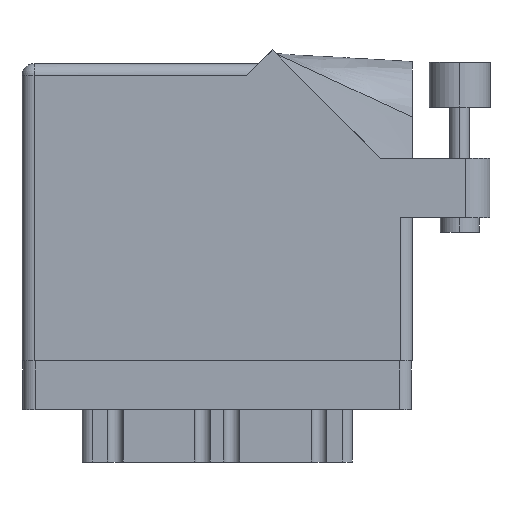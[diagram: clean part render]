
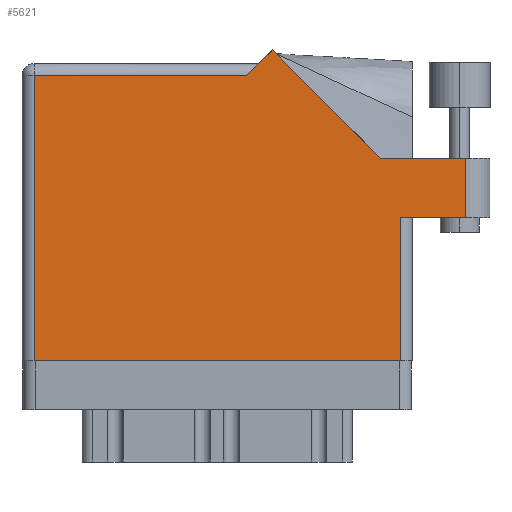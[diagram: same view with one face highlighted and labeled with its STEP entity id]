
A CAD part, front view. The second image highlights one B-rep face of the part: STEP entity #5621.
In plain terms, the highlighted face is planar.
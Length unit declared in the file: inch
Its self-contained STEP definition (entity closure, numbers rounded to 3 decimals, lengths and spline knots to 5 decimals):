
#240 = EDGE_CURVE ( 'NONE', #29193, #4980, #17073, .T. ) ;
#394 = EDGE_CURVE ( 'NONE', #23292, #6392, #9847, .T. ) ;
#606 = VERTEX_POINT ( 'NONE', #11222 ) ;
#652 = DIRECTION ( 'NONE',  ( 0., -1., 0. ) ) ;
#1379 = VECTOR ( 'NONE', #17937, 39.37008 ) ;
#1610 = DIRECTION ( 'NONE',  ( -1., 0., 0. ) ) ;
#2080 = CARTESIAN_POINT ( 'NONE',  ( 1.28771, 1.60071, 0. ) ) ;
#2123 = CARTESIAN_POINT ( 'NONE',  ( 0., 1.468, 0. ) ) ;
#2800 = ORIENTED_EDGE ( 'NONE', *, *, #3490, .T. ) ;
#3029 = ORIENTED_EDGE ( 'NONE', *, *, #5789, .T. ) ;
#3490 = EDGE_CURVE ( 'NONE', #606, #23292, #8045, .T. ) ;
#4129 = VERTEX_POINT ( 'NONE', #16466 ) ;
#4789 = CARTESIAN_POINT ( 'NONE',  ( 0., 1.53, 0. ) ) ;
#4980 = VERTEX_POINT ( 'NONE', #5910 ) ;
#5215 = CARTESIAN_POINT ( 'NONE',  ( 2.285, 1.044, 0. ) ) ;
#5621 = ADVANCED_FACE ( 'NONE', ( #32142 ), #34264, .F. ) ;
#5724 = EDGE_CURVE ( 'NONE', #6392, #8947, #15922, .T. ) ;
#5789 = EDGE_CURVE ( 'NONE', #26999, #606, #16603, .T. ) ;
#5910 = CARTESIAN_POINT ( 'NONE',  ( 1.948, 0., 0. ) ) ;
#6138 = EDGE_CURVE ( 'NONE', #4980, #26999, #32280, .T. ) ;
#6392 = VERTEX_POINT ( 'NONE', #25359 ) ;
#6677 = CARTESIAN_POINT ( 'NONE',  ( 2.285, 1.044, 0. ) ) ;
#7183 = CARTESIAN_POINT ( 'NONE',  ( 2.41, 1.044, 0. ) ) ;
#8045 = LINE ( 'NONE', #5215, #26473 ) ;
#8100 = DIRECTION ( 'NONE',  ( 0., 1., 0. ) ) ;
#8370 = ORIENTED_EDGE ( 'NONE', *, *, #6138, .T. ) ;
#8484 = CARTESIAN_POINT ( 'NONE',  ( 1.84442, 1.044, 0. ) ) ;
#8761 = VECTOR ( 'NONE', #8100, 39.37008 ) ;
#8947 = VERTEX_POINT ( 'NONE', #2080 ) ;
#9288 = CARTESIAN_POINT ( 'NONE',  ( 1.948, 0.737, 0. ) ) ;
#9847 = LINE ( 'NONE', #7183, #1379 ) ;
#10406 = VERTEX_POINT ( 'NONE', #27486 ) ;
#11044 = DIRECTION ( 'NONE',  ( 0., 1., 0. ) ) ;
#11222 = CARTESIAN_POINT ( 'NONE',  ( 2.285, 0.737, 0. ) ) ;
#11412 = LINE ( 'NONE', #21975, #34405 ) ;
#12050 = ORIENTED_EDGE ( 'NONE', *, *, #19920, .T. ) ;
#12279 = EDGE_LOOP ( 'NONE', ( #3029, #2800, #31864, #31094, #23018, #12050, #18805, #20165, #8370 ) ) ;
#12758 = LINE ( 'NONE', #2123, #33790 ) ;
#13274 = CARTESIAN_POINT ( 'NONE',  ( 0., 0., 0. ) ) ;
#13916 = LINE ( 'NONE', #32779, #26219 ) ;
#14462 = AXIS2_PLACEMENT_3D ( 'NONE', #4789, #16093, #34450 ) ;
#15922 = LINE ( 'NONE', #8484, #17833 ) ;
#16093 = DIRECTION ( 'NONE',  ( 0., 0., -1. ) ) ;
#16466 = CARTESIAN_POINT ( 'NONE',  ( 1.155, 1.468, 0. ) ) ;
#16603 = LINE ( 'NONE', #27521, #20105 ) ;
#16894 = DIRECTION ( 'NONE',  ( 1., 0., 0. ) ) ;
#17073 = LINE ( 'NONE', #13274, #17742 ) ;
#17742 = VECTOR ( 'NONE', #16894, 39.37008 ) ;
#17833 = VECTOR ( 'NONE', #30179, 39.37008 ) ;
#17937 = DIRECTION ( 'NONE',  ( -1., 0., 0. ) ) ;
#18805 = ORIENTED_EDGE ( 'NONE', *, *, #31655, .T. ) ;
#19920 = EDGE_CURVE ( 'NONE', #4129, #10406, #12758, .T. ) ;
#20105 = VECTOR ( 'NONE', #22066, 39.37008 ) ;
#20165 = ORIENTED_EDGE ( 'NONE', *, *, #240, .T. ) ;
#21975 = CARTESIAN_POINT ( 'NONE',  ( 1.217, 1.53, 0. ) ) ;
#22066 = DIRECTION ( 'NONE',  ( 1., 0., 0. ) ) ;
#23018 = ORIENTED_EDGE ( 'NONE', *, *, #25516, .T. ) ;
#23292 = VERTEX_POINT ( 'NONE', #6677 ) ;
#23462 = CARTESIAN_POINT ( 'NONE',  ( 1.948, 0.737, 0. ) ) ;
#24282 = DIRECTION ( 'NONE',  ( -0.707, -0.707, 0. ) ) ;
#25359 = CARTESIAN_POINT ( 'NONE',  ( 1.84442, 1.044, 0. ) ) ;
#25516 = EDGE_CURVE ( 'NONE', #8947, #4129, #11412, .T. ) ;
#26219 = VECTOR ( 'NONE', #652, 39.37008 ) ;
#26473 = VECTOR ( 'NONE', #11044, 39.37008 ) ;
#26999 = VERTEX_POINT ( 'NONE', #9288 ) ;
#27486 = CARTESIAN_POINT ( 'NONE',  ( 0.062, 1.468, 0. ) ) ;
#27521 = CARTESIAN_POINT ( 'NONE',  ( 2.01, 0.737, 0. ) ) ;
#29193 = VERTEX_POINT ( 'NONE', #34756 ) ;
#30179 = DIRECTION ( 'NONE',  ( -0.707, 0.707, 0. ) ) ;
#31094 = ORIENTED_EDGE ( 'NONE', *, *, #5724, .T. ) ;
#31655 = EDGE_CURVE ( 'NONE', #10406, #29193, #13916, .T. ) ;
#31864 = ORIENTED_EDGE ( 'NONE', *, *, #394, .T. ) ;
#32142 = FACE_OUTER_BOUND ( 'NONE', #12279, .T. ) ;
#32280 = LINE ( 'NONE', #23462, #8761 ) ;
#32779 = CARTESIAN_POINT ( 'NONE',  ( 0.062, 0., 0. ) ) ;
#33790 = VECTOR ( 'NONE', #1610, 39.37008 ) ;
#34264 = PLANE ( 'NONE',  #14462 ) ;
#34405 = VECTOR ( 'NONE', #24282, 39.37008 ) ;
#34450 = DIRECTION ( 'NONE',  ( -1., 0., 0. ) ) ;
#34756 = CARTESIAN_POINT ( 'NONE',  ( 0.062, 0., 0. ) ) ;
